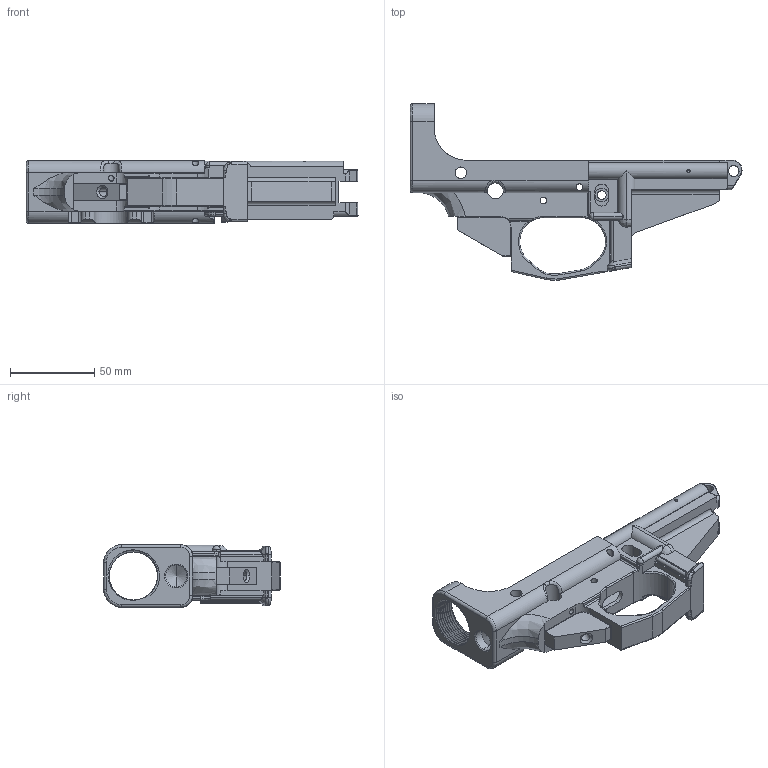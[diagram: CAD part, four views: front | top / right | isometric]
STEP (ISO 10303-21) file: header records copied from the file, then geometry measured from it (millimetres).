
FILE_DESCRIPTION (( 'STEP AP214' ), '1' );
FILE_NAME ('Single_Shot_Lower.STEP', '2013-10-23T01:32:50', ( '' ), ( '' ), 'SwSTEP 2.0', 'SolidWorks 2013', '' );
FILE_SCHEMA (( 'AUTOMOTIVE_DESIGN' ));
Length unit declared in the file: inch
Products named in the file (1): Single_Shot_Lower
Bounding box: 197.08 x 104.92 x 37.13 mm (x, y, z)
Volume: 162736.9 mm3; surface area: 48140.7 mm2
Topology: 2 solids, 2 shells, 596 faces, 1628 edges, 1030 vertices
Faces by surface type: cylinder 230, plane 223, bspline 131, cone 12
Entity records: 43746 total; most frequent: CARTESIAN_POINT 29872, ORIENTED_EDGE 3230, DIRECTION 2453, EDGE_CURVE 1615, VERTEX_POINT 1030, VECTOR 835, LINE 835, AXIS2_PLACEMENT_3D 809
